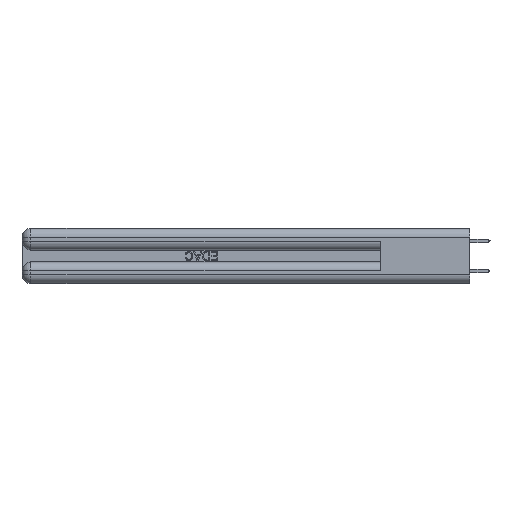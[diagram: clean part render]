
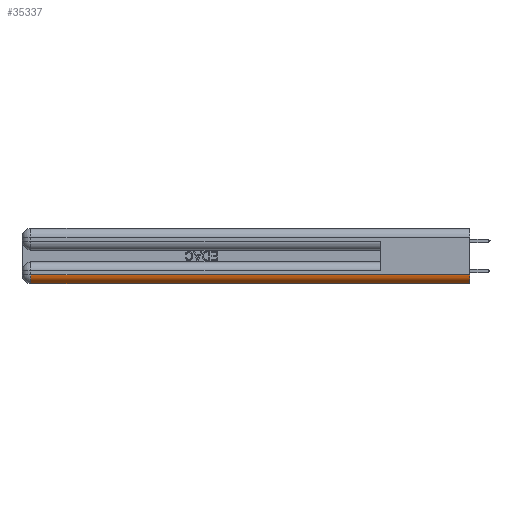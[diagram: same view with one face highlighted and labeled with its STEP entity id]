
A CAD part, left-side view. The second image highlights one B-rep face of the part: STEP entity #35337.
In plain terms, the highlighted cylindrical face has radius 1.524 mm (diameter 3.048 mm), a partial arc.
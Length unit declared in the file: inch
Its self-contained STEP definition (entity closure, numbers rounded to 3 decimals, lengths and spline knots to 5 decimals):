
#2027 = DIRECTION ( 'NONE',  ( 0., 0., 1. ) ) ;
#2905 = AXIS2_PLACEMENT_3D ( 'NONE', #34444, #23650, #38171 ) ;
#3974 = DIRECTION ( 'NONE',  ( 0., 0., 1. ) ) ;
#4387 = CARTESIAN_POINT ( 'NONE',  ( 0., 0., 0.06 ) ) ;
#5112 = AXIS2_PLACEMENT_3D ( 'NONE', #18669, #11731, #3974 ) ;
#8776 = VECTOR ( 'NONE', #25925, 39.37008 ) ;
#10666 = VERTEX_POINT ( 'NONE', #23769 ) ;
#11731 = DIRECTION ( 'NONE',  ( 0., 1., 0. ) ) ;
#12911 = ORIENTED_EDGE ( 'NONE', *, *, #46079, .F. ) ;
#14345 = LINE ( 'NONE', #4387, #42683 ) ;
#14346 = ORIENTED_EDGE ( 'NONE', *, *, #30221, .F. ) ;
#14839 = CARTESIAN_POINT ( 'NONE',  ( 0.06, 3., 0. ) ) ;
#14986 = CARTESIAN_POINT ( 'NONE',  ( 0., 0., 0.06 ) ) ;
#16496 = CYLINDRICAL_SURFACE ( 'NONE', #5112, 0.06 ) ;
#18159 = CIRCLE ( 'NONE', #2905, 0.06 ) ;
#18669 = CARTESIAN_POINT ( 'NONE',  ( 0.06, 0., 0.06 ) ) ;
#20920 = LINE ( 'NONE', #14839, #8776 ) ;
#21128 = FACE_OUTER_BOUND ( 'NONE', #35962, .T. ) ;
#21251 = CIRCLE ( 'NONE', #32486, 0.06 ) ;
#22819 = DIRECTION ( 'NONE',  ( 0., -1., 0. ) ) ;
#23650 = DIRECTION ( 'NONE',  ( 0., 1., 0. ) ) ;
#23769 = CARTESIAN_POINT ( 'NONE',  ( 0.06, 2.94, 0. ) ) ;
#24223 = DIRECTION ( 'NONE',  ( 0., -1., 0. ) ) ;
#25925 = DIRECTION ( 'NONE',  ( 0., 1., 0. ) ) ;
#26645 = VERTEX_POINT ( 'NONE', #30100 ) ;
#30100 = CARTESIAN_POINT ( 'NONE',  ( 0.06, 0., 0. ) ) ;
#30221 = EDGE_CURVE ( 'NONE', #30996, #26645, #21251, .T. ) ;
#30335 = VERTEX_POINT ( 'NONE', #43478 ) ;
#30996 = VERTEX_POINT ( 'NONE', #14986 ) ;
#31014 = EDGE_CURVE ( 'NONE', #26645, #10666, #20920, .T. ) ;
#31462 = ORIENTED_EDGE ( 'NONE', *, *, #31014, .F. ) ;
#32486 = AXIS2_PLACEMENT_3D ( 'NONE', #35183, #24223, #2027 ) ;
#34172 = EDGE_CURVE ( 'NONE', #30335, #30996, #14345, .T. ) ;
#34444 = CARTESIAN_POINT ( 'NONE',  ( 0.06, 2.94, 0.06 ) ) ;
#35183 = CARTESIAN_POINT ( 'NONE',  ( 0.06, 0., 0.06 ) ) ;
#35337 = ADVANCED_FACE ( 'NONE', ( #21128 ), #16496, .T. ) ;
#35962 = EDGE_LOOP ( 'NONE', ( #14346, #43782, #12911, #31462 ) ) ;
#38171 = DIRECTION ( 'NONE',  ( 0., 0., 1. ) ) ;
#42683 = VECTOR ( 'NONE', #22819, 39.37008 ) ;
#43478 = CARTESIAN_POINT ( 'NONE',  ( 0., 2.94, 0.06 ) ) ;
#43782 = ORIENTED_EDGE ( 'NONE', *, *, #34172, .F. ) ;
#46079 = EDGE_CURVE ( 'NONE', #10666, #30335, #18159, .T. ) ;
